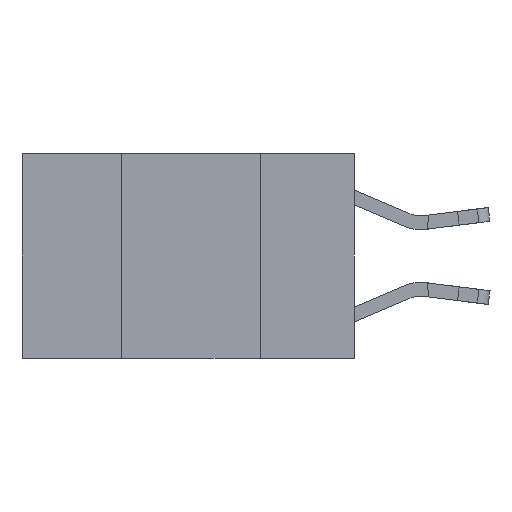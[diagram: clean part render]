
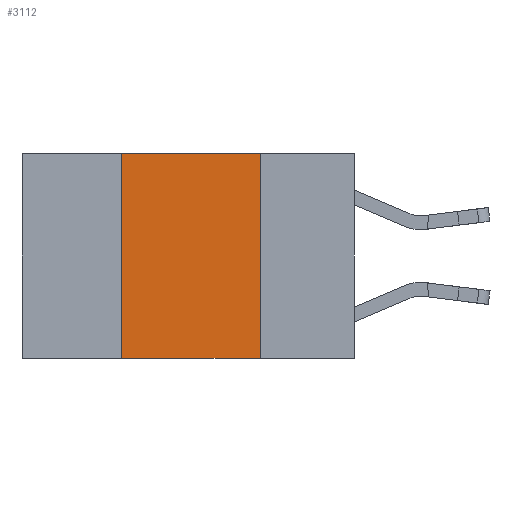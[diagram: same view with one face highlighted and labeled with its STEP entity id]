
A CAD part, left-side view. The second image highlights one B-rep face of the part: STEP entity #3112.
In plain terms, the highlighted planar face has unit normal (-1, 0, 0).
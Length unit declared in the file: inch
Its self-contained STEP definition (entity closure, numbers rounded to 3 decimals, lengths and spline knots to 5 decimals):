
#269 = DIRECTION ( 'NONE',  ( 1., 0., 0. ) ) ;
#332 = FACE_OUTER_BOUND ( 'NONE', #10343, .T. ) ;
#395 = CARTESIAN_POINT ( 'NONE',  ( 0., 0.42, -0.37 ) ) ;
#501 = DIRECTION ( 'NONE',  ( 0., -1., 0. ) ) ;
#697 = CARTESIAN_POINT ( 'NONE',  ( 0., 0.17, 0. ) ) ;
#1059 = CARTESIAN_POINT ( 'NONE',  ( 0., 0.42, 0. ) ) ;
#1234 = VERTEX_POINT ( 'NONE', #395 ) ;
#1447 = LINE ( 'NONE', #4755, #12015 ) ;
#1855 = LINE ( 'NONE', #5300, #12371 ) ;
#2618 = ORIENTED_EDGE ( 'NONE', *, *, #9342, .T. ) ;
#2664 = EDGE_CURVE ( 'NONE', #4271, #10666, #3665, .T. ) ;
#2919 = VERTEX_POINT ( 'NONE', #1059 ) ;
#3112 = ADVANCED_FACE ( 'NONE', ( #332 ), #6660, .F. ) ;
#3615 = CARTESIAN_POINT ( 'NONE',  ( 0., 0.6, 0. ) ) ;
#3665 = LINE ( 'NONE', #697, #8861 ) ;
#4271 = VERTEX_POINT ( 'NONE', #9578 ) ;
#4755 = CARTESIAN_POINT ( 'NONE',  ( 0., 0.6, -0.37 ) ) ;
#5127 = LINE ( 'NONE', #3615, #12867 ) ;
#5300 = CARTESIAN_POINT ( 'NONE',  ( 0., 0.42, 0. ) ) ;
#6218 = AXIS2_PLACEMENT_3D ( 'NONE', #12619, #269, #7712 ) ;
#6660 = PLANE ( 'NONE',  #6218 ) ;
#7712 = DIRECTION ( 'NONE',  ( 0., 0., -1. ) ) ;
#8087 = ORIENTED_EDGE ( 'NONE', *, *, #11307, .F. ) ;
#8861 = VECTOR ( 'NONE', #12063, 39.37008 ) ;
#8878 = ORIENTED_EDGE ( 'NONE', *, *, #10060, .F. ) ;
#9342 = EDGE_CURVE ( 'NONE', #1234, #10666, #1447, .T. ) ;
#9578 = CARTESIAN_POINT ( 'NONE',  ( 0., 0.17, 0. ) ) ;
#10060 = EDGE_CURVE ( 'NONE', #2919, #4271, #5127, .T. ) ;
#10221 = ORIENTED_EDGE ( 'NONE', *, *, #2664, .F. ) ;
#10343 = EDGE_LOOP ( 'NONE', ( #10221, #8878, #8087, #2618 ) ) ;
#10443 = DIRECTION ( 'NONE',  ( 0., 0., 1. ) ) ;
#10599 = CARTESIAN_POINT ( 'NONE',  ( 0., 0.17, -0.37 ) ) ;
#10666 = VERTEX_POINT ( 'NONE', #10599 ) ;
#11307 = EDGE_CURVE ( 'NONE', #1234, #2919, #1855, .T. ) ;
#12015 = VECTOR ( 'NONE', #501, 39.37008 ) ;
#12063 = DIRECTION ( 'NONE',  ( 0., 0., -1. ) ) ;
#12371 = VECTOR ( 'NONE', #10443, 39.37008 ) ;
#12619 = CARTESIAN_POINT ( 'NONE',  ( 0., 0.6, 0. ) ) ;
#12756 = DIRECTION ( 'NONE',  ( 0., -1., 0. ) ) ;
#12867 = VECTOR ( 'NONE', #12756, 39.37008 ) ;
